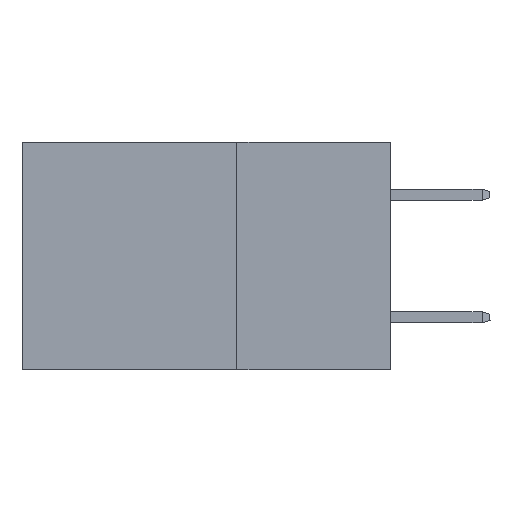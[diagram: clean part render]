
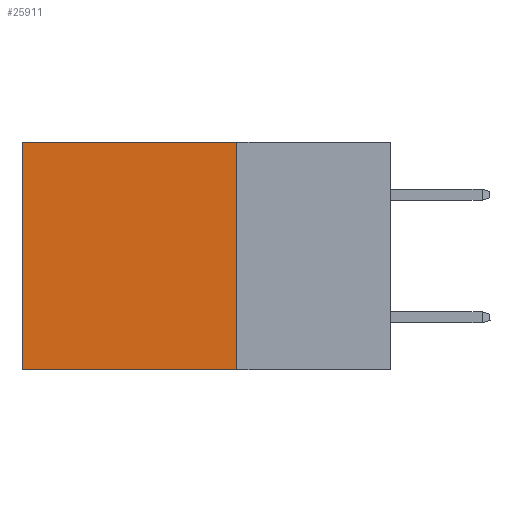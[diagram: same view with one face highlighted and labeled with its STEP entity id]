
A CAD part, left-side view. The second image highlights one B-rep face of the part: STEP entity #25911.
In plain terms, the highlighted planar face has unit normal (-1, 0, 0).
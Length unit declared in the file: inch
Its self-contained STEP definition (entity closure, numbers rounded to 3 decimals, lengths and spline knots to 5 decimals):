
#3889 = LINE ( 'NONE', #10657, #16296 ) ;
#4396 = DIRECTION ( 'NONE',  ( 1., 0., 0. ) ) ;
#5669 = EDGE_CURVE ( 'NONE', #26499, #32407, #25536, .T. ) ;
#6176 = VERTEX_POINT ( 'NONE', #15046 ) ;
#7854 = VERTEX_POINT ( 'NONE', #29485 ) ;
#10657 = CARTESIAN_POINT ( 'NONE',  ( 0.2875, 0.25, 0. ) ) ;
#10752 = VECTOR ( 'NONE', #35238, 39.37008 ) ;
#11876 = DIRECTION ( 'NONE',  ( 0., 0., -1. ) ) ;
#12777 = ORIENTED_EDGE ( 'NONE', *, *, #31072, .T. ) ;
#15046 = CARTESIAN_POINT ( 'NONE',  ( 0.2875, 0.6, -0.37 ) ) ;
#15499 = PLANE ( 'NONE',  #19738 ) ;
#16296 = VECTOR ( 'NONE', #18866, 39.37008 ) ;
#16563 = ORIENTED_EDGE ( 'NONE', *, *, #5669, .F. ) ;
#18866 = DIRECTION ( 'NONE',  ( 0., 1., 0. ) ) ;
#19738 = AXIS2_PLACEMENT_3D ( 'NONE', #37509, #4396, #11876 ) ;
#22152 = DIRECTION ( 'NONE',  ( 0., 0., -1. ) ) ;
#25536 = LINE ( 'NONE', #40314, #32600 ) ;
#25911 = ADVANCED_FACE ( 'NONE', ( #29999 ), #15499, .F. ) ;
#26499 = VERTEX_POINT ( 'NONE', #26556 ) ;
#26556 = CARTESIAN_POINT ( 'NONE',  ( 0.2875, 0.25, 0. ) ) ;
#27730 = CARTESIAN_POINT ( 'NONE',  ( 0.2875, 0.6, 0. ) ) ;
#27901 = LINE ( 'NONE', #42917, #42689 ) ;
#29485 = CARTESIAN_POINT ( 'NONE',  ( 0.2875, 0.6, 0. ) ) ;
#29999 = FACE_OUTER_BOUND ( 'NONE', #41159, .T. ) ;
#30554 = ORIENTED_EDGE ( 'NONE', *, *, #37935, .T. ) ;
#31072 = EDGE_CURVE ( 'NONE', #7854, #6176, #46627, .T. ) ;
#32407 = VERTEX_POINT ( 'NONE', #36219 ) ;
#32600 = VECTOR ( 'NONE', #22152, 39.37008 ) ;
#35238 = DIRECTION ( 'NONE',  ( 0., 0., -1. ) ) ;
#36219 = CARTESIAN_POINT ( 'NONE',  ( 0.2875, 0.25, -0.37 ) ) ;
#37509 = CARTESIAN_POINT ( 'NONE',  ( 0.2875, 0.25, 0. ) ) ;
#37935 = EDGE_CURVE ( 'NONE', #26499, #7854, #3889, .T. ) ;
#39028 = EDGE_CURVE ( 'NONE', #32407, #6176, #27901, .T. ) ;
#40250 = ORIENTED_EDGE ( 'NONE', *, *, #39028, .F. ) ;
#40314 = CARTESIAN_POINT ( 'NONE',  ( 0.2875, 0.25, 0. ) ) ;
#41159 = EDGE_LOOP ( 'NONE', ( #12777, #40250, #16563, #30554 ) ) ;
#42685 = DIRECTION ( 'NONE',  ( 0., 1., 0. ) ) ;
#42689 = VECTOR ( 'NONE', #42685, 39.37008 ) ;
#42917 = CARTESIAN_POINT ( 'NONE',  ( 0.2875, 0.25, -0.37 ) ) ;
#46627 = LINE ( 'NONE', #27730, #10752 ) ;
